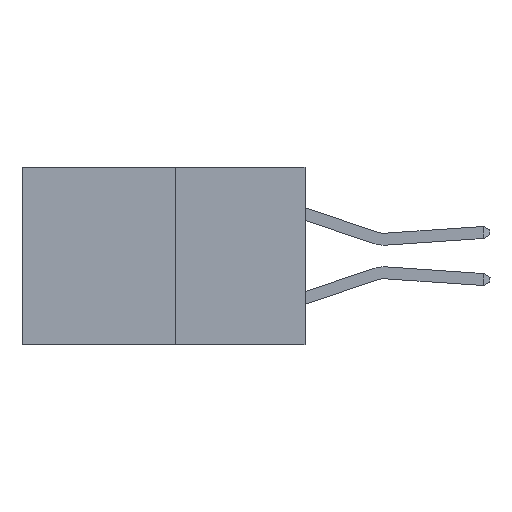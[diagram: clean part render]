
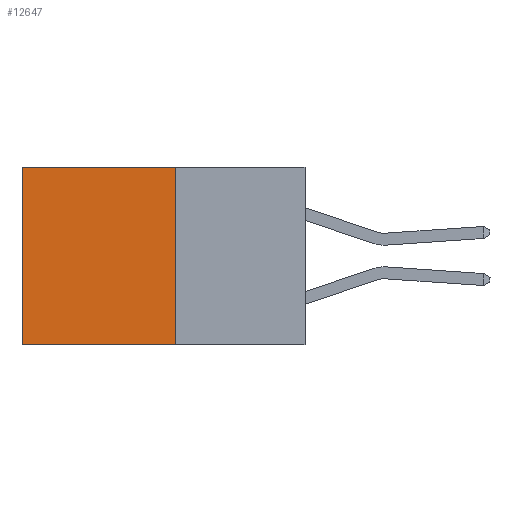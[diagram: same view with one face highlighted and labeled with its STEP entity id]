
A CAD part, left-side view. The second image highlights one B-rep face of the part: STEP entity #12647.
In plain terms, the highlighted planar face has unit normal (-1, 0, 0).
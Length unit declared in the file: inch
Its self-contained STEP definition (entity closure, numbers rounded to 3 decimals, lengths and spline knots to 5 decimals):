
#257 = CARTESIAN_POINT ( 'NONE',  ( 0.277, 0.27, -0.37 ) ) ;
#2496 = EDGE_LOOP ( 'NONE', ( #21490, #13403, #24874, #14586 ) ) ;
#3259 = PLANE ( 'NONE',  #16671 ) ;
#3624 = VECTOR ( 'NONE', #26196, 39.37008 ) ;
#3686 = CARTESIAN_POINT ( 'NONE',  ( 0.277, 0.59, -0.37 ) ) ;
#3767 = VECTOR ( 'NONE', #26872, 39.37008 ) ;
#3865 = VERTEX_POINT ( 'NONE', #18116 ) ;
#4024 = LINE ( 'NONE', #3686, #16304 ) ;
#6217 = DIRECTION ( 'NONE',  ( 0., 0., -1. ) ) ;
#6858 = CARTESIAN_POINT ( 'NONE',  ( 0.277, 0.27, -0.37 ) ) ;
#8282 = DIRECTION ( 'NONE',  ( 0., 0., -1. ) ) ;
#12647 = ADVANCED_FACE ( 'NONE', ( #20166 ), #3259, .F. ) ;
#13403 = ORIENTED_EDGE ( 'NONE', *, *, #22004, .F. ) ;
#14308 = CARTESIAN_POINT ( 'NONE',  ( 0.277, 0.27, 0. ) ) ;
#14586 = ORIENTED_EDGE ( 'NONE', *, *, #20673, .T. ) ;
#14925 = LINE ( 'NONE', #6858, #15662 ) ;
#15401 = CARTESIAN_POINT ( 'NONE',  ( 0.277, 0.27, -0.37 ) ) ;
#15662 = VECTOR ( 'NONE', #23766, 39.37008 ) ;
#15840 = VERTEX_POINT ( 'NONE', #29359 ) ;
#16304 = VECTOR ( 'NONE', #6217, 39.37008 ) ;
#16671 = AXIS2_PLACEMENT_3D ( 'NONE', #20282, #22722, #8282 ) ;
#17838 = EDGE_CURVE ( 'NONE', #31132, #17932, #29443, .T. ) ;
#17932 = VERTEX_POINT ( 'NONE', #15401 ) ;
#18116 = CARTESIAN_POINT ( 'NONE',  ( 0.277, 0.59, 0. ) ) ;
#20166 = FACE_OUTER_BOUND ( 'NONE', #2496, .T. ) ;
#20282 = CARTESIAN_POINT ( 'NONE',  ( 0.277, 0.27, -0.37 ) ) ;
#20673 = EDGE_CURVE ( 'NONE', #31132, #3865, #23024, .T. ) ;
#21490 = ORIENTED_EDGE ( 'NONE', *, *, #28527, .T. ) ;
#22004 = EDGE_CURVE ( 'NONE', #17932, #15840, #14925, .T. ) ;
#22722 = DIRECTION ( 'NONE',  ( 1., 0., 0. ) ) ;
#23024 = LINE ( 'NONE', #14308, #3624 ) ;
#23766 = DIRECTION ( 'NONE',  ( 0., 1., 0. ) ) ;
#24874 = ORIENTED_EDGE ( 'NONE', *, *, #17838, .F. ) ;
#26196 = DIRECTION ( 'NONE',  ( 0., 1., 0. ) ) ;
#26872 = DIRECTION ( 'NONE',  ( 0., 0., -1. ) ) ;
#28154 = CARTESIAN_POINT ( 'NONE',  ( 0.277, 0.27, 0. ) ) ;
#28527 = EDGE_CURVE ( 'NONE', #3865, #15840, #4024, .T. ) ;
#29359 = CARTESIAN_POINT ( 'NONE',  ( 0.277, 0.59, -0.37 ) ) ;
#29443 = LINE ( 'NONE', #257, #3767 ) ;
#31132 = VERTEX_POINT ( 'NONE', #28154 ) ;
